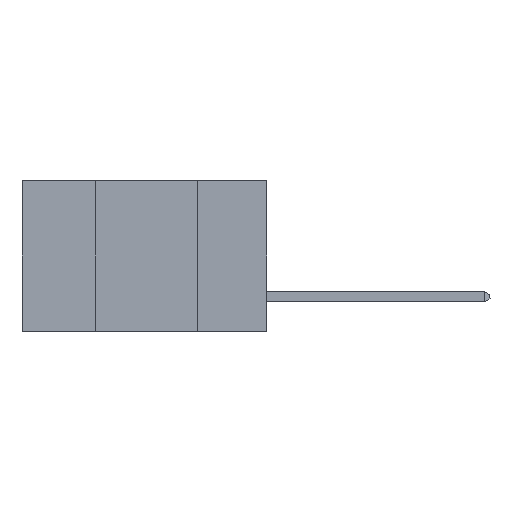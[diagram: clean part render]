
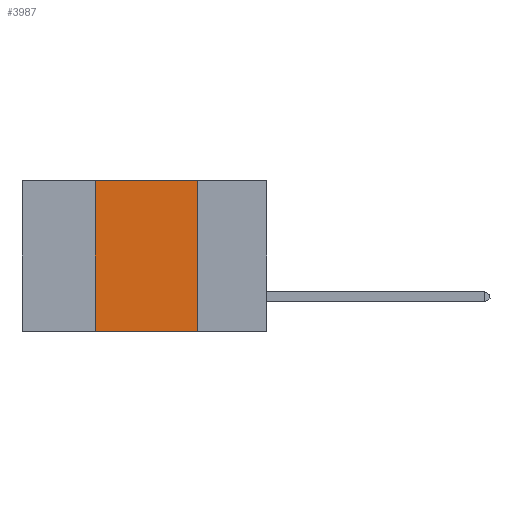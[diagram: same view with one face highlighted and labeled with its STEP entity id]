
A CAD part, left-side view. The second image highlights one B-rep face of the part: STEP entity #3987.
In plain terms, the highlighted planar face has unit normal (-1, 0, 0).
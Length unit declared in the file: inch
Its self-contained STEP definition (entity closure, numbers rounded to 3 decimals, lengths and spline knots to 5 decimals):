
#317 = DIRECTION ( 'NONE',  ( 0., 0., -1. ) ) ;
#496 = DIRECTION ( 'NONE',  ( 0., 0., 1. ) ) ;
#509 = DIRECTION ( 'NONE',  ( 0., 0., -1. ) ) ;
#693 = LINE ( 'NONE', #8937, #5598 ) ;
#826 = EDGE_CURVE ( 'NONE', #10794, #4547, #8754, .T. ) ;
#2063 = ORIENTED_EDGE ( 'NONE', *, *, #826, .T. ) ;
#3018 = CARTESIAN_POINT ( 'NONE',  ( 0., 0.42, -0.37 ) ) ;
#3117 = CARTESIAN_POINT ( 'NONE',  ( 0., 0.17, -0.37 ) ) ;
#3444 = VECTOR ( 'NONE', #9998, 39.37008 ) ;
#3470 = EDGE_CURVE ( 'NONE', #10794, #7681, #693, .T. ) ;
#3536 = VECTOR ( 'NONE', #10434, 39.37008 ) ;
#3987 = ADVANCED_FACE ( 'NONE', ( #7618 ), #5174, .F. ) ;
#4282 = CARTESIAN_POINT ( 'NONE',  ( 0., 0.42, 0. ) ) ;
#4547 = VERTEX_POINT ( 'NONE', #3117 ) ;
#4583 = ORIENTED_EDGE ( 'NONE', *, *, #4751, .F. ) ;
#4751 = EDGE_CURVE ( 'NONE', #4839, #4547, #11220, .T. ) ;
#4839 = VERTEX_POINT ( 'NONE', #10795 ) ;
#4896 = EDGE_CURVE ( 'NONE', #7681, #4839, #10415, .T. ) ;
#5174 = PLANE ( 'NONE',  #5633 ) ;
#5403 = ORIENTED_EDGE ( 'NONE', *, *, #3470, .F. ) ;
#5421 = CARTESIAN_POINT ( 'NONE',  ( 0., 0.17, 0. ) ) ;
#5598 = VECTOR ( 'NONE', #496, 39.37008 ) ;
#5633 = AXIS2_PLACEMENT_3D ( 'NONE', #7921, #6173, #317 ) ;
#6173 = DIRECTION ( 'NONE',  ( 1., 0., 0. ) ) ;
#6317 = ORIENTED_EDGE ( 'NONE', *, *, #4896, .F. ) ;
#7203 = VECTOR ( 'NONE', #509, 39.37008 ) ;
#7618 = FACE_OUTER_BOUND ( 'NONE', #11626, .T. ) ;
#7681 = VERTEX_POINT ( 'NONE', #4282 ) ;
#7921 = CARTESIAN_POINT ( 'NONE',  ( 0., 0.6, 0. ) ) ;
#8754 = LINE ( 'NONE', #10531, #3536 ) ;
#8937 = CARTESIAN_POINT ( 'NONE',  ( 0., 0.42, 0. ) ) ;
#9998 = DIRECTION ( 'NONE',  ( 0., -1., 0. ) ) ;
#10415 = LINE ( 'NONE', #11733, #3444 ) ;
#10434 = DIRECTION ( 'NONE',  ( 0., -1., 0. ) ) ;
#10531 = CARTESIAN_POINT ( 'NONE',  ( 0., 0.6, -0.37 ) ) ;
#10794 = VERTEX_POINT ( 'NONE', #3018 ) ;
#10795 = CARTESIAN_POINT ( 'NONE',  ( 0., 0.17, 0. ) ) ;
#11220 = LINE ( 'NONE', #5421, #7203 ) ;
#11626 = EDGE_LOOP ( 'NONE', ( #4583, #6317, #5403, #2063 ) ) ;
#11733 = CARTESIAN_POINT ( 'NONE',  ( 0., 0.6, 0. ) ) ;
